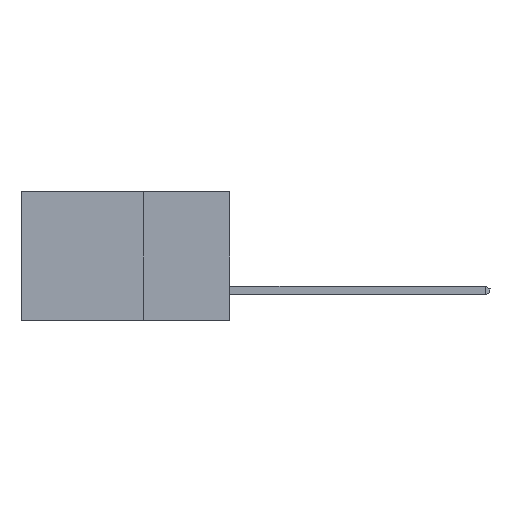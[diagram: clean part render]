
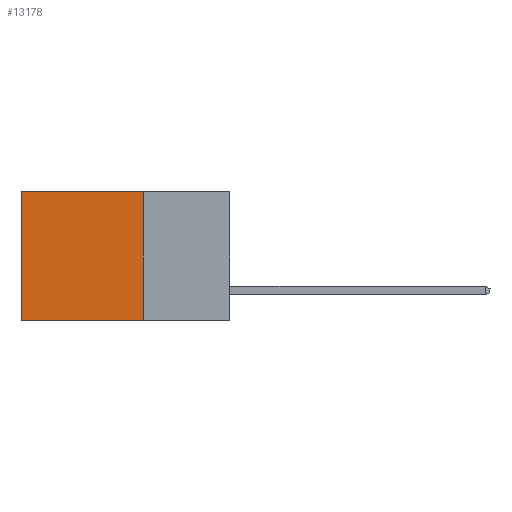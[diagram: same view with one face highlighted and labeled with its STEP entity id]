
A CAD part, left-side view. The second image highlights one B-rep face of the part: STEP entity #13178.
In plain terms, the highlighted planar face has unit normal (-1, 0, 0).
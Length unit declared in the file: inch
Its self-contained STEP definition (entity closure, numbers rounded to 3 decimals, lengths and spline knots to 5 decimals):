
#69 = AXIS2_PLACEMENT_3D ( 'NONE', #11051, #9652, #15409 ) ;
#302 = CARTESIAN_POINT ( 'NONE',  ( 0.2615, 0.25, -0.37 ) ) ;
#454 = ORIENTED_EDGE ( 'NONE', *, *, #9100, .T. ) ;
#1273 = VECTOR ( 'NONE', #14746, 39.37008 ) ;
#1438 = LINE ( 'NONE', #4260, #12712 ) ;
#1450 = EDGE_CURVE ( 'NONE', #14484, #15156, #10410, .T. ) ;
#1875 = LINE ( 'NONE', #2068, #6559 ) ;
#2068 = CARTESIAN_POINT ( 'NONE',  ( 0.2615, 0.25, 0. ) ) ;
#2254 = DIRECTION ( 'NONE',  ( 0., 1., 0. ) ) ;
#2763 = VERTEX_POINT ( 'NONE', #7252 ) ;
#3291 = ORIENTED_EDGE ( 'NONE', *, *, #16745, .T. ) ;
#3627 = CARTESIAN_POINT ( 'NONE',  ( 0.2615, 0.25, -0.37 ) ) ;
#3719 = DIRECTION ( 'NONE',  ( 0., 0., -1. ) ) ;
#4260 = CARTESIAN_POINT ( 'NONE',  ( 0.2615, 0.6, -0.37 ) ) ;
#6503 = ORIENTED_EDGE ( 'NONE', *, *, #1450, .F. ) ;
#6559 = VECTOR ( 'NONE', #2254, 39.37008 ) ;
#7252 = CARTESIAN_POINT ( 'NONE',  ( 0.2615, 0.6, 0. ) ) ;
#7560 = EDGE_CURVE ( 'NONE', #10156, #14484, #10914, .T. ) ;
#8017 = CARTESIAN_POINT ( 'NONE',  ( 0.2615, 0.6, -0.37 ) ) ;
#8472 = CARTESIAN_POINT ( 'NONE',  ( 0.2615, 0.25, 0. ) ) ;
#9100 = EDGE_CURVE ( 'NONE', #10156, #2763, #1875, .T. ) ;
#9652 = DIRECTION ( 'NONE',  ( 1., 0., 0. ) ) ;
#10156 = VERTEX_POINT ( 'NONE', #8472 ) ;
#10224 = CARTESIAN_POINT ( 'NONE',  ( 0.2615, 0.25, -0.37 ) ) ;
#10410 = LINE ( 'NONE', #10224, #1273 ) ;
#10914 = LINE ( 'NONE', #3627, #14774 ) ;
#11051 = CARTESIAN_POINT ( 'NONE',  ( 0.2615, 0.25, -0.37 ) ) ;
#12712 = VECTOR ( 'NONE', #12865, 39.37008 ) ;
#12826 = ORIENTED_EDGE ( 'NONE', *, *, #7560, .F. ) ;
#12865 = DIRECTION ( 'NONE',  ( 0., 0., -1. ) ) ;
#13178 = ADVANCED_FACE ( 'NONE', ( #16720 ), #18180, .F. ) ;
#14484 = VERTEX_POINT ( 'NONE', #302 ) ;
#14746 = DIRECTION ( 'NONE',  ( 0., 1., 0. ) ) ;
#14774 = VECTOR ( 'NONE', #3719, 39.37008 ) ;
#14967 = EDGE_LOOP ( 'NONE', ( #3291, #6503, #12826, #454 ) ) ;
#15156 = VERTEX_POINT ( 'NONE', #8017 ) ;
#15409 = DIRECTION ( 'NONE',  ( 0., 0., -1. ) ) ;
#16720 = FACE_OUTER_BOUND ( 'NONE', #14967, .T. ) ;
#16745 = EDGE_CURVE ( 'NONE', #2763, #15156, #1438, .T. ) ;
#18180 = PLANE ( 'NONE',  #69 ) ;
